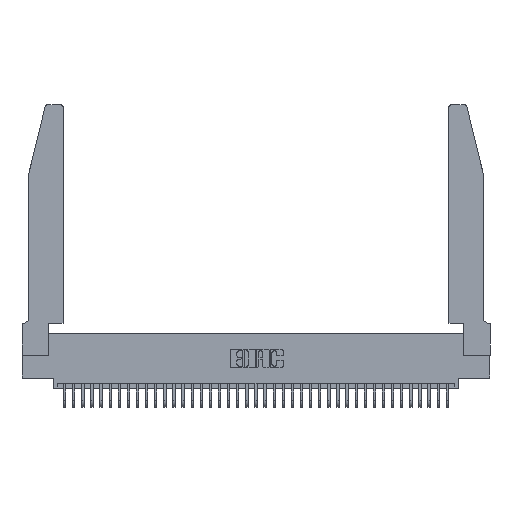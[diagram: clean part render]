
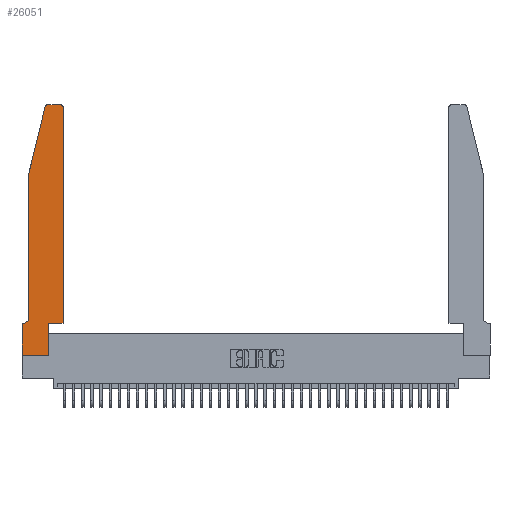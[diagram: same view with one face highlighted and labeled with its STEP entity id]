
A CAD part, top view. The second image highlights one B-rep face of the part: STEP entity #26051.
In plain terms, the highlighted planar face has unit normal (0, 0, 1).
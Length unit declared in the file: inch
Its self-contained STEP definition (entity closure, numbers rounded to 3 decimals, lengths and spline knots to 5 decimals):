
#290 = CARTESIAN_POINT ( 'NONE',  ( 0.4505, 2.72, 0.37 ) ) ;
#299 = CARTESIAN_POINT ( 'NONE',  ( 0.0755, 2., 0.37 ) ) ;
#591 = DIRECTION ( 'NONE',  ( 0., -1., 0. ) ) ;
#617 = VERTEX_POINT ( 'NONE', #16910 ) ;
#781 = VERTEX_POINT ( 'NONE', #290 ) ;
#869 = ORIENTED_EDGE ( 'NONE', *, *, #17980, .T. ) ;
#1265 = DIRECTION ( 'NONE',  ( 1., 0., 0. ) ) ;
#1753 = AXIS2_PLACEMENT_3D ( 'NONE', #2160, #24107, #5401 ) ;
#2139 = ORIENTED_EDGE ( 'NONE', *, *, #27233, .T. ) ;
#2160 = CARTESIAN_POINT ( 'NONE',  ( 0.284, 2.72, 0.37 ) ) ;
#2252 = LINE ( 'NONE', #13962, #34282 ) ;
#2394 = EDGE_CURVE ( 'NONE', #617, #23188, #5996, .T. ) ;
#2852 = PLANE ( 'NONE',  #29009 ) ;
#4167 = ORIENTED_EDGE ( 'NONE', *, *, #15482, .T. ) ;
#4969 = LINE ( 'NONE', #36196, #28833 ) ;
#5194 = CARTESIAN_POINT ( 'NONE',  ( 0.0755, 2., 0.37 ) ) ;
#5401 = DIRECTION ( 'NONE',  ( 1., 0., 0. ) ) ;
#5547 = LINE ( 'NONE', #299, #36435 ) ;
#5832 = VERTEX_POINT ( 'NONE', #39611 ) ;
#5847 = CARTESIAN_POINT ( 'NONE',  ( 0.0055, 0.42, 0.37 ) ) ;
#5918 = VECTOR ( 'NONE', #11633, 39.37008 ) ;
#5996 = LINE ( 'NONE', #20108, #37823 ) ;
#6089 = DIRECTION ( 'NONE',  ( 0., 0., 1. ) ) ;
#6268 = VERTEX_POINT ( 'NONE', #29310 ) ;
#6287 = EDGE_CURVE ( 'NONE', #29098, #20362, #2252, .T. ) ;
#7192 = EDGE_CURVE ( 'NONE', #6268, #5832, #35703, .T. ) ;
#8144 = DIRECTION ( 'NONE',  ( 0., 0., 1. ) ) ;
#9079 = DIRECTION ( 'NONE',  ( -1., 0., 0. ) ) ;
#10622 = ORIENTED_EDGE ( 'NONE', *, *, #2394, .T. ) ;
#11011 = EDGE_CURVE ( 'NONE', #20362, #617, #13514, .T. ) ;
#11355 = VERTEX_POINT ( 'NONE', #23314 ) ;
#11633 = DIRECTION ( 'NONE',  ( -1., 0., 0. ) ) ;
#11815 = DIRECTION ( 'NONE',  ( 0., 1., 0. ) ) ;
#11905 = CARTESIAN_POINT ( 'NONE',  ( 0.4505, 0.35, 0.37 ) ) ;
#12218 = VECTOR ( 'NONE', #12945, 39.37008 ) ;
#12552 = EDGE_CURVE ( 'NONE', #781, #6268, #14832, .T. ) ;
#12711 = ORIENTED_EDGE ( 'NONE', *, *, #6287, .T. ) ;
#12945 = DIRECTION ( 'NONE',  ( -1., 0., 0. ) ) ;
#13514 = LINE ( 'NONE', #18751, #28965 ) ;
#13962 = CARTESIAN_POINT ( 'NONE',  ( 0., 0., 0.37 ) ) ;
#14832 = CIRCLE ( 'NONE', #25382, 0.03 ) ;
#15267 = LINE ( 'NONE', #36022, #5918 ) ;
#15482 = EDGE_CURVE ( 'NONE', #11355, #17004, #24835, .T. ) ;
#15553 = CARTESIAN_POINT ( 'NONE',  ( 0., 0., 0.37 ) ) ;
#16123 = CIRCLE ( 'NONE', #1753, 0.03 ) ;
#16225 = LINE ( 'NONE', #37466, #17181 ) ;
#16910 = CARTESIAN_POINT ( 'NONE',  ( 0.2865, 0.35, 0.37 ) ) ;
#16941 = ORIENTED_EDGE ( 'NONE', *, *, #7192, .T. ) ;
#17004 = VERTEX_POINT ( 'NONE', #35553 ) ;
#17181 = VECTOR ( 'NONE', #19242, 39.37008 ) ;
#17183 = EDGE_CURVE ( 'NONE', #23188, #781, #4969, .T. ) ;
#17980 = EDGE_CURVE ( 'NONE', #34744, #29098, #16225, .T. ) ;
#18751 = CARTESIAN_POINT ( 'NONE',  ( 0.2865, 0.35, 0.37 ) ) ;
#19242 = DIRECTION ( 'NONE',  ( 0., -1., 0. ) ) ;
#20108 = CARTESIAN_POINT ( 'NONE',  ( 0.4505, 0.35, 0.37 ) ) ;
#20362 = VERTEX_POINT ( 'NONE', #22919 ) ;
#20731 = ORIENTED_EDGE ( 'NONE', *, *, #17183, .T. ) ;
#21674 = CARTESIAN_POINT ( 'NONE',  ( 0., 0.35, 0.37 ) ) ;
#22822 = VERTEX_POINT ( 'NONE', #28819 ) ;
#22919 = CARTESIAN_POINT ( 'NONE',  ( 0.2865, 0., 0.37 ) ) ;
#23188 = VERTEX_POINT ( 'NONE', #11905 ) ;
#23314 = CARTESIAN_POINT ( 'NONE',  ( 0.25487, 2.72718, 0.37 ) ) ;
#24107 = DIRECTION ( 'NONE',  ( 0., 0., 1. ) ) ;
#24398 = ORIENTED_EDGE ( 'NONE', *, *, #11011, .T. ) ;
#24779 = CARTESIAN_POINT ( 'NONE',  ( 0., 0.35, 0.37 ) ) ;
#24835 = LINE ( 'NONE', #5194, #31952 ) ;
#25229 = CIRCLE ( 'NONE', #28769, 0.07 ) ;
#25382 = AXIS2_PLACEMENT_3D ( 'NONE', #26747, #8144, #29794 ) ;
#25895 = EDGE_CURVE ( 'NONE', #5832, #11355, #16123, .T. ) ;
#26051 = ADVANCED_FACE ( 'NONE', ( #26757 ), #2852, .T. ) ;
#26276 = CARTESIAN_POINT ( 'NONE',  ( 0.0755, 0.42, 0.37 ) ) ;
#26299 = DIRECTION ( 'NONE',  ( 1., 0., 0. ) ) ;
#26747 = CARTESIAN_POINT ( 'NONE',  ( 0.4205, 2.72, 0.37 ) ) ;
#26757 = FACE_OUTER_BOUND ( 'NONE', #35395, .T. ) ;
#26888 = ORIENTED_EDGE ( 'NONE', *, *, #25895, .T. ) ;
#27233 = EDGE_CURVE ( 'NONE', #39488, #22822, #25229, .T. ) ;
#27625 = DIRECTION ( 'NONE',  ( 0., 0., -1. ) ) ;
#27848 = DIRECTION ( 'NONE',  ( 1., 0., 0. ) ) ;
#28769 = AXIS2_PLACEMENT_3D ( 'NONE', #5847, #27625, #9079 ) ;
#28819 = CARTESIAN_POINT ( 'NONE',  ( 0.0055, 0.35, 0.37 ) ) ;
#28833 = VECTOR ( 'NONE', #11815, 39.37008 ) ;
#28965 = VECTOR ( 'NONE', #40030, 39.37008 ) ;
#29009 = AXIS2_PLACEMENT_3D ( 'NONE', #24779, #6089, #27848 ) ;
#29098 = VERTEX_POINT ( 'NONE', #15553 ) ;
#29255 = ORIENTED_EDGE ( 'NONE', *, *, #36250, .T. ) ;
#29310 = CARTESIAN_POINT ( 'NONE',  ( 0.4205, 2.75, 0.37 ) ) ;
#29794 = DIRECTION ( 'NONE',  ( 1., 0., 0. ) ) ;
#30049 = DIRECTION ( 'NONE',  ( -0.239, -0.971, 0. ) ) ;
#31362 = CARTESIAN_POINT ( 'NONE',  ( 0.2605, 2.75, 0.37 ) ) ;
#31952 = VECTOR ( 'NONE', #30049, 39.37008 ) ;
#34282 = VECTOR ( 'NONE', #1265, 39.37008 ) ;
#34744 = VERTEX_POINT ( 'NONE', #21674 ) ;
#35395 = EDGE_LOOP ( 'NONE', ( #16941, #26888, #4167, #29255, #2139, #36414, #869, #12711, #24398, #10622, #20731, #35575 ) ) ;
#35553 = CARTESIAN_POINT ( 'NONE',  ( 0.0755, 2., 0.37 ) ) ;
#35575 = ORIENTED_EDGE ( 'NONE', *, *, #12552, .T. ) ;
#35703 = LINE ( 'NONE', #31362, #12218 ) ;
#36022 = CARTESIAN_POINT ( 'NONE',  ( 0.0755, 0.35, 0.37 ) ) ;
#36196 = CARTESIAN_POINT ( 'NONE',  ( 0.4505, 0.35, 0.37 ) ) ;
#36250 = EDGE_CURVE ( 'NONE', #17004, #39488, #5547, .T. ) ;
#36414 = ORIENTED_EDGE ( 'NONE', *, *, #37792, .T. ) ;
#36435 = VECTOR ( 'NONE', #591, 39.37008 ) ;
#37466 = CARTESIAN_POINT ( 'NONE',  ( 0., 0., 0.37 ) ) ;
#37792 = EDGE_CURVE ( 'NONE', #22822, #34744, #15267, .T. ) ;
#37823 = VECTOR ( 'NONE', #26299, 39.37008 ) ;
#39488 = VERTEX_POINT ( 'NONE', #26276 ) ;
#39611 = CARTESIAN_POINT ( 'NONE',  ( 0.284, 2.75, 0.37 ) ) ;
#40030 = DIRECTION ( 'NONE',  ( 0., 1., 0. ) ) ;
